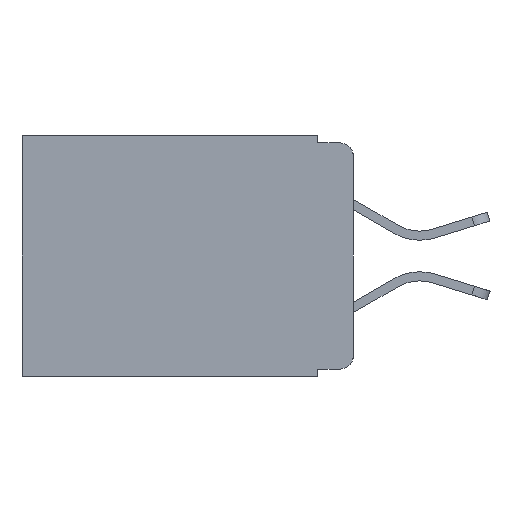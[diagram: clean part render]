
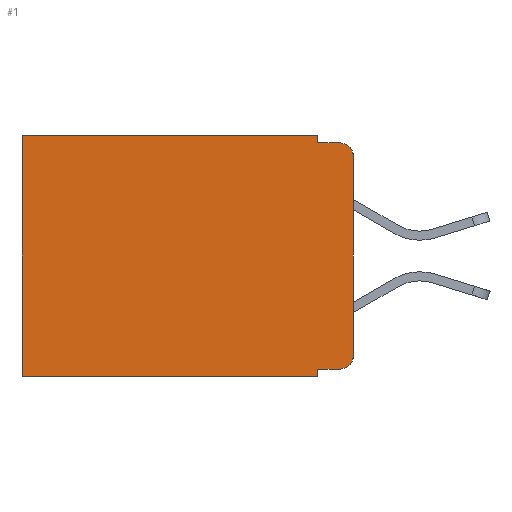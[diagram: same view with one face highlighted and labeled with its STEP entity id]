
A CAD part, left-side view. The second image highlights one B-rep face of the part: STEP entity #1.
In plain terms, the highlighted planar face has unit normal (-1, 0, 0).
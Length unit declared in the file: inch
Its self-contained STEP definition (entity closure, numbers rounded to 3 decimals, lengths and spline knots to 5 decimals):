
#1 = ADVANCED_FACE ( 'NONE', ( #7730 ), #710, .F. ) ;
#22 = CARTESIAN_POINT ( 'NONE',  ( 0.298, 0.051, -0.333 ) ) ;
#501 = LINE ( 'NONE', #12397, #4941 ) ;
#581 = VERTEX_POINT ( 'NONE', #13521 ) ;
#710 = PLANE ( 'NONE',  #4632 ) ;
#960 = DIRECTION ( 'NONE',  ( 0., 0., -1. ) ) ;
#1015 = VERTEX_POINT ( 'NONE', #5666 ) ;
#1743 = CARTESIAN_POINT ( 'NONE',  ( 0.298, 0.051, 0. ) ) ;
#1772 = VERTEX_POINT ( 'NONE', #6825 ) ;
#1829 = EDGE_CURVE ( 'NONE', #1772, #581, #12068, .T. ) ;
#1913 = VECTOR ( 'NONE', #9350, 39.37008 ) ;
#2132 = DIRECTION ( 'NONE',  ( 0., -1., 0. ) ) ;
#2657 = LINE ( 'NONE', #8770, #15018 ) ;
#2723 = ORIENTED_EDGE ( 'NONE', *, *, #1829, .F. ) ;
#2732 = LINE ( 'NONE', #3161, #1913 ) ;
#2989 = EDGE_CURVE ( 'NONE', #1015, #6644, #501, .T. ) ;
#3048 = VERTEX_POINT ( 'NONE', #22 ) ;
#3161 = CARTESIAN_POINT ( 'NONE',  ( 0.298, 0.473, 0. ) ) ;
#3348 = CARTESIAN_POINT ( 'NONE',  ( 0.298, 0., 0. ) ) ;
#3383 = CARTESIAN_POINT ( 'NONE',  ( 0.298, 0., 0. ) ) ;
#3657 = CARTESIAN_POINT ( 'NONE',  ( 0.298, 0.02, -0.01 ) ) ;
#4209 = DIRECTION ( 'NONE',  ( -1., 0., 0. ) ) ;
#4604 = DIRECTION ( 'NONE',  ( 1., 0., 0. ) ) ;
#4632 = AXIS2_PLACEMENT_3D ( 'NONE', #3348, #4604, #12266 ) ;
#4694 = CARTESIAN_POINT ( 'NONE',  ( 0.298, 0.473, -0.343 ) ) ;
#4702 = LINE ( 'NONE', #9793, #13633 ) ;
#4912 = ORIENTED_EDGE ( 'NONE', *, *, #9215, .T. ) ;
#4929 = LINE ( 'NONE', #6658, #8454 ) ;
#4941 = VECTOR ( 'NONE', #6120, 39.37008 ) ;
#5666 = CARTESIAN_POINT ( 'NONE',  ( 0.298, 0.051, 0. ) ) ;
#5825 = VERTEX_POINT ( 'NONE', #6743 ) ;
#5938 = ORIENTED_EDGE ( 'NONE', *, *, #12528, .F. ) ;
#6099 = EDGE_CURVE ( 'NONE', #5825, #10610, #15390, .T. ) ;
#6120 = DIRECTION ( 'NONE',  ( 0., 0., -1. ) ) ;
#6644 = VERTEX_POINT ( 'NONE', #11173 ) ;
#6658 = CARTESIAN_POINT ( 'NONE',  ( 0.298, 0.051, -0.333 ) ) ;
#6743 = CARTESIAN_POINT ( 'NONE',  ( 0.298, 0.051, -0.343 ) ) ;
#6825 = CARTESIAN_POINT ( 'NONE',  ( 0.298, 0., -0.03 ) ) ;
#7301 = EDGE_CURVE ( 'NONE', #15896, #581, #9986, .T. ) ;
#7375 = DIRECTION ( 'NONE',  ( 0., 1., 0. ) ) ;
#7520 = AXIS2_PLACEMENT_3D ( 'NONE', #14337, #4209, #8223 ) ;
#7730 = FACE_OUTER_BOUND ( 'NONE', #8392, .T. ) ;
#7855 = VECTOR ( 'NONE', #13493, 39.37008 ) ;
#8223 = DIRECTION ( 'NONE',  ( 0., 0., -1. ) ) ;
#8392 = EDGE_LOOP ( 'NONE', ( #2723, #4912, #5938, #9837, #14717, #8965, #11798, #14741, #9674, #15746 ) ) ;
#8454 = VECTOR ( 'NONE', #10467, 39.37008 ) ;
#8600 = CARTESIAN_POINT ( 'NONE',  ( 0.298, 0.02, -0.03 ) ) ;
#8770 = CARTESIAN_POINT ( 'NONE',  ( 0.298, 0., 0. ) ) ;
#8874 = EDGE_CURVE ( 'NONE', #13637, #10610, #2732, .T. ) ;
#8965 = ORIENTED_EDGE ( 'NONE', *, *, #8874, .T. ) ;
#9215 = EDGE_CURVE ( 'NONE', #1772, #14013, #11501, .T. ) ;
#9350 = DIRECTION ( 'NONE',  ( 0., 0., -1. ) ) ;
#9674 = ORIENTED_EDGE ( 'NONE', *, *, #10900, .T. ) ;
#9678 = CARTESIAN_POINT ( 'NONE',  ( 0.298, 0.473, 0. ) ) ;
#9793 = CARTESIAN_POINT ( 'NONE',  ( 0.298, 0.051, -0.01 ) ) ;
#9837 = ORIENTED_EDGE ( 'NONE', *, *, #2989, .F. ) ;
#9986 = CIRCLE ( 'NONE', #7520, 0.02 ) ;
#10467 = DIRECTION ( 'NONE',  ( 0., -1., 0. ) ) ;
#10550 = LINE ( 'NONE', #1743, #15898 ) ;
#10610 = VERTEX_POINT ( 'NONE', #4694 ) ;
#10900 = EDGE_CURVE ( 'NONE', #3048, #15896, #4929, .T. ) ;
#11173 = CARTESIAN_POINT ( 'NONE',  ( 0.298, 0.051, -0.01 ) ) ;
#11501 = CIRCLE ( 'NONE', #14238, 0.02 ) ;
#11798 = ORIENTED_EDGE ( 'NONE', *, *, #6099, .F. ) ;
#12068 = LINE ( 'NONE', #3383, #7855 ) ;
#12266 = DIRECTION ( 'NONE',  ( 0., 0., -1. ) ) ;
#12397 = CARTESIAN_POINT ( 'NONE',  ( 0.298, 0.051, 0. ) ) ;
#12528 = EDGE_CURVE ( 'NONE', #6644, #14013, #4702, .T. ) ;
#12812 = EDGE_CURVE ( 'NONE', #1015, #13637, #2657, .T. ) ;
#13493 = DIRECTION ( 'NONE',  ( 0., 0., -1. ) ) ;
#13521 = CARTESIAN_POINT ( 'NONE',  ( 0.298, 0., -0.313 ) ) ;
#13633 = VECTOR ( 'NONE', #2132, 39.37008 ) ;
#13637 = VERTEX_POINT ( 'NONE', #9678 ) ;
#13809 = DIRECTION ( 'NONE',  ( 0., 1., 0. ) ) ;
#14013 = VERTEX_POINT ( 'NONE', #3657 ) ;
#14238 = AXIS2_PLACEMENT_3D ( 'NONE', #8600, #16229, #960 ) ;
#14337 = CARTESIAN_POINT ( 'NONE',  ( 0.298, 0.02, -0.313 ) ) ;
#14717 = ORIENTED_EDGE ( 'NONE', *, *, #12812, .T. ) ;
#14741 = ORIENTED_EDGE ( 'NONE', *, *, #15647, .F. ) ;
#14772 = VECTOR ( 'NONE', #13809, 39.37008 ) ;
#15012 = CARTESIAN_POINT ( 'NONE',  ( 0.298, 0.02, -0.333 ) ) ;
#15018 = VECTOR ( 'NONE', #7375, 39.37008 ) ;
#15390 = LINE ( 'NONE', #16257, #14772 ) ;
#15569 = DIRECTION ( 'NONE',  ( 0., 0., -1. ) ) ;
#15647 = EDGE_CURVE ( 'NONE', #3048, #5825, #10550, .T. ) ;
#15746 = ORIENTED_EDGE ( 'NONE', *, *, #7301, .T. ) ;
#15896 = VERTEX_POINT ( 'NONE', #15012 ) ;
#15898 = VECTOR ( 'NONE', #15569, 39.37008 ) ;
#16229 = DIRECTION ( 'NONE',  ( -1., 0., 0. ) ) ;
#16257 = CARTESIAN_POINT ( 'NONE',  ( 0.298, 0., -0.343 ) ) ;
